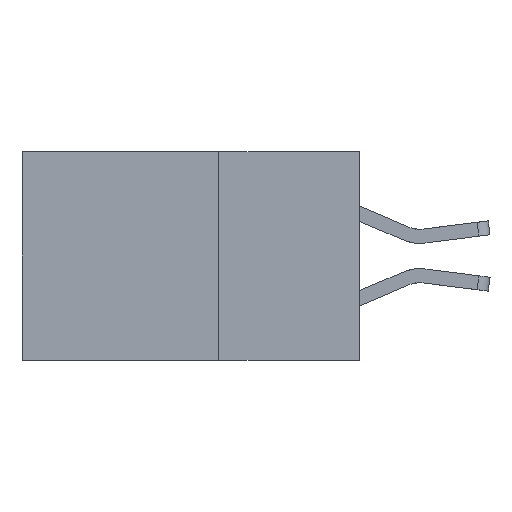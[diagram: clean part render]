
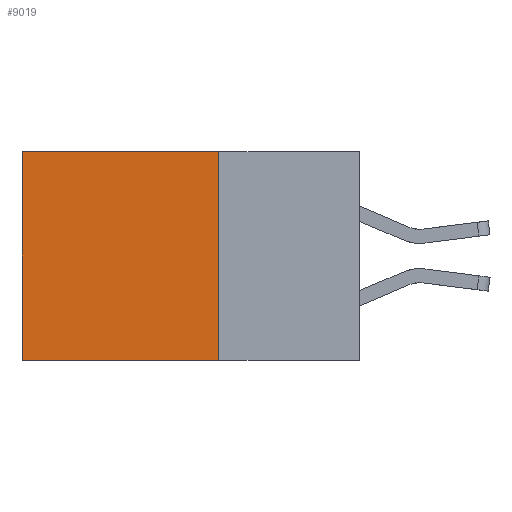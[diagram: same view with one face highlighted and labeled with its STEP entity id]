
A CAD part, left-side view. The second image highlights one B-rep face of the part: STEP entity #9019.
In plain terms, the highlighted planar face has unit normal (-1, 0, 0).
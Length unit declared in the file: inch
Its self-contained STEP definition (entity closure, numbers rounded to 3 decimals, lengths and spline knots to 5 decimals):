
#60 = CARTESIAN_POINT ( 'NONE',  ( 0.2875, 0.25, 0. ) ) ;
#212 = CARTESIAN_POINT ( 'NONE',  ( 0.2875, 0.6, 0. ) ) ;
#335 = VERTEX_POINT ( 'NONE', #7132 ) ;
#672 = DIRECTION ( 'NONE',  ( 0., 1., 0. ) ) ;
#758 = EDGE_CURVE ( 'NONE', #5231, #9232, #6782, .T. ) ;
#1364 = CARTESIAN_POINT ( 'NONE',  ( 0.2875, 0.6, 0. ) ) ;
#1526 = DIRECTION ( 'NONE',  ( 1., 0., 0. ) ) ;
#1953 = EDGE_CURVE ( 'NONE', #335, #7838, #5651, .T. ) ;
#2077 = LINE ( 'NONE', #1364, #8849 ) ;
#2230 = LINE ( 'NONE', #2401, #8335 ) ;
#2289 = DIRECTION ( 'NONE',  ( 0., 1., 0. ) ) ;
#2329 = CARTESIAN_POINT ( 'NONE',  ( 0.2875, 0.6, -0.37 ) ) ;
#2353 = CARTESIAN_POINT ( 'NONE',  ( 0.2875, 0.25, -0.37 ) ) ;
#2401 = CARTESIAN_POINT ( 'NONE',  ( 0.2875, 0.25, 0. ) ) ;
#3643 = EDGE_CURVE ( 'NONE', #5231, #335, #2230, .T. ) ;
#3771 = CARTESIAN_POINT ( 'NONE',  ( 0.2875, 0.25, 0. ) ) ;
#4135 = EDGE_LOOP ( 'NONE', ( #7077, #4514, #6272, #4366 ) ) ;
#4165 = FACE_OUTER_BOUND ( 'NONE', #4135, .T. ) ;
#4366 = ORIENTED_EDGE ( 'NONE', *, *, #758, .T. ) ;
#4514 = ORIENTED_EDGE ( 'NONE', *, *, #1953, .F. ) ;
#5011 = DIRECTION ( 'NONE',  ( 0., 0., -1. ) ) ;
#5231 = VERTEX_POINT ( 'NONE', #3771 ) ;
#5438 = VECTOR ( 'NONE', #2289, 39.37008 ) ;
#5516 = CARTESIAN_POINT ( 'NONE',  ( 0.2875, 0.25, 0. ) ) ;
#5651 = LINE ( 'NONE', #2353, #5438 ) ;
#6272 = ORIENTED_EDGE ( 'NONE', *, *, #3643, .F. ) ;
#6495 = PLANE ( 'NONE',  #7226 ) ;
#6525 = DIRECTION ( 'NONE',  ( 0., 0., -1. ) ) ;
#6713 = EDGE_CURVE ( 'NONE', #9232, #7838, #2077, .T. ) ;
#6782 = LINE ( 'NONE', #5516, #8433 ) ;
#7077 = ORIENTED_EDGE ( 'NONE', *, *, #6713, .T. ) ;
#7132 = CARTESIAN_POINT ( 'NONE',  ( 0.2875, 0.25, -0.37 ) ) ;
#7226 = AXIS2_PLACEMENT_3D ( 'NONE', #60, #1526, #6525 ) ;
#7361 = DIRECTION ( 'NONE',  ( 0., 0., -1. ) ) ;
#7838 = VERTEX_POINT ( 'NONE', #2329 ) ;
#8335 = VECTOR ( 'NONE', #7361, 39.37008 ) ;
#8433 = VECTOR ( 'NONE', #672, 39.37008 ) ;
#8849 = VECTOR ( 'NONE', #5011, 39.37008 ) ;
#9019 = ADVANCED_FACE ( 'NONE', ( #4165 ), #6495, .F. ) ;
#9232 = VERTEX_POINT ( 'NONE', #212 ) ;
